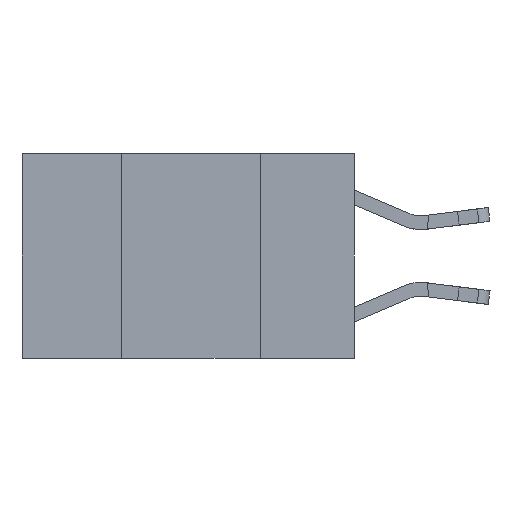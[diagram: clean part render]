
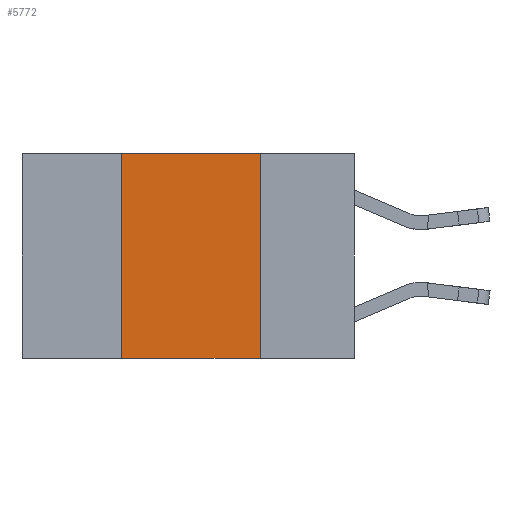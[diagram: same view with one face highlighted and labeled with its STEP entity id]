
A CAD part, left-side view. The second image highlights one B-rep face of the part: STEP entity #5772.
In plain terms, the highlighted planar face has unit normal (-1, 0, 0).
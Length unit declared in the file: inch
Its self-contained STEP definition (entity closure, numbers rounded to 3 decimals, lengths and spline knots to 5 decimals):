
#957 = CARTESIAN_POINT ( 'NONE',  ( 0., 0.6, 0. ) ) ;
#1206 = CARTESIAN_POINT ( 'NONE',  ( 0., 0.17, 0. ) ) ;
#1589 = CARTESIAN_POINT ( 'NONE',  ( 0., 0.6, 0. ) ) ;
#1845 = ORIENTED_EDGE ( 'NONE', *, *, #15746, .F. ) ;
#2154 = VERTEX_POINT ( 'NONE', #6644 ) ;
#2545 = DIRECTION ( 'NONE',  ( 0., 0., -1. ) ) ;
#4389 = LINE ( 'NONE', #1589, #15644 ) ;
#5158 = CARTESIAN_POINT ( 'NONE',  ( 0., 0.42, -0.37 ) ) ;
#5532 = FACE_OUTER_BOUND ( 'NONE', #16968, .T. ) ;
#5713 = LINE ( 'NONE', #7379, #14466 ) ;
#5772 = ADVANCED_FACE ( 'NONE', ( #5532 ), #10092, .F. ) ;
#5907 = ORIENTED_EDGE ( 'NONE', *, *, #14328, .F. ) ;
#6644 = CARTESIAN_POINT ( 'NONE',  ( 0., 0.17, 0. ) ) ;
#7379 = CARTESIAN_POINT ( 'NONE',  ( 0., 0.42, 0. ) ) ;
#8426 = VERTEX_POINT ( 'NONE', #5158 ) ;
#9164 = DIRECTION ( 'NONE',  ( 0., -1., 0. ) ) ;
#9518 = EDGE_CURVE ( 'NONE', #8426, #13677, #5713, .T. ) ;
#9936 = ORIENTED_EDGE ( 'NONE', *, *, #9518, .F. ) ;
#10092 = PLANE ( 'NONE',  #12769 ) ;
#10129 = CARTESIAN_POINT ( 'NONE',  ( 0., 0.42, 0. ) ) ;
#11569 = DIRECTION ( 'NONE',  ( 1., 0., 0. ) ) ;
#11786 = DIRECTION ( 'NONE',  ( 0., 0., -1. ) ) ;
#12391 = LINE ( 'NONE', #12621, #15695 ) ;
#12468 = EDGE_CURVE ( 'NONE', #8426, #13470, #12391, .T. ) ;
#12621 = CARTESIAN_POINT ( 'NONE',  ( 0., 0.6, -0.37 ) ) ;
#12769 = AXIS2_PLACEMENT_3D ( 'NONE', #957, #11569, #2545 ) ;
#13470 = VERTEX_POINT ( 'NONE', #16895 ) ;
#13677 = VERTEX_POINT ( 'NONE', #10129 ) ;
#14043 = DIRECTION ( 'NONE',  ( 0., -1., 0. ) ) ;
#14209 = ORIENTED_EDGE ( 'NONE', *, *, #12468, .T. ) ;
#14328 = EDGE_CURVE ( 'NONE', #13677, #2154, #4389, .T. ) ;
#14466 = VECTOR ( 'NONE', #16134, 39.37008 ) ;
#15644 = VECTOR ( 'NONE', #9164, 39.37008 ) ;
#15695 = VECTOR ( 'NONE', #14043, 39.37008 ) ;
#15746 = EDGE_CURVE ( 'NONE', #2154, #13470, #16692, .T. ) ;
#16134 = DIRECTION ( 'NONE',  ( 0., 0., 1. ) ) ;
#16278 = VECTOR ( 'NONE', #11786, 39.37008 ) ;
#16692 = LINE ( 'NONE', #1206, #16278 ) ;
#16895 = CARTESIAN_POINT ( 'NONE',  ( 0., 0.17, -0.37 ) ) ;
#16968 = EDGE_LOOP ( 'NONE', ( #1845, #5907, #9936, #14209 ) ) ;
